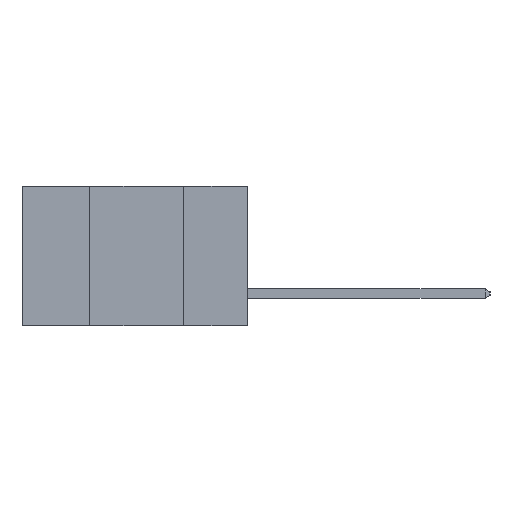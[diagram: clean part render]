
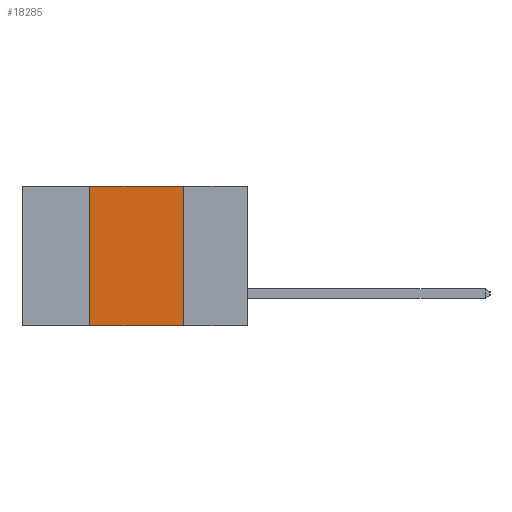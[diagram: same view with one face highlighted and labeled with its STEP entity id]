
A CAD part, left-side view. The second image highlights one B-rep face of the part: STEP entity #18285.
In plain terms, the highlighted planar face has unit normal (-1, 0, 0).
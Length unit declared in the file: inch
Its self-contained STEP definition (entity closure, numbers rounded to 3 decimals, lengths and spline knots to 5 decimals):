
#1420 = VERTEX_POINT ( 'NONE', #10792 ) ;
#1421 = CARTESIAN_POINT ( 'NONE',  ( 0., 0.42, 0. ) ) ;
#1899 = CARTESIAN_POINT ( 'NONE',  ( 0., 0.17, 0. ) ) ;
#2328 = EDGE_CURVE ( 'NONE', #19285, #11708, #9535, .T. ) ;
#3021 = AXIS2_PLACEMENT_3D ( 'NONE', #13472, #15572, #3329 ) ;
#3329 = DIRECTION ( 'NONE',  ( 0., 0., -1. ) ) ;
#4172 = VECTOR ( 'NONE', #22159, 39.37008 ) ;
#4933 = CARTESIAN_POINT ( 'NONE',  ( 0., 0.17, 0. ) ) ;
#5813 = FACE_OUTER_BOUND ( 'NONE', #22244, .T. ) ;
#6110 = VECTOR ( 'NONE', #19828, 39.37008 ) ;
#7272 = CARTESIAN_POINT ( 'NONE',  ( 0., 0.42, 0. ) ) ;
#9337 = DIRECTION ( 'NONE',  ( 0., 0., 1. ) ) ;
#9535 = LINE ( 'NONE', #1899, #4172 ) ;
#10020 = LINE ( 'NONE', #26420, #14842 ) ;
#10792 = CARTESIAN_POINT ( 'NONE',  ( 0., 0.42, -0.37 ) ) ;
#11410 = PLANE ( 'NONE',  #3021 ) ;
#11708 = VERTEX_POINT ( 'NONE', #19326 ) ;
#12136 = DIRECTION ( 'NONE',  ( 0., -1., 0. ) ) ;
#12950 = ORIENTED_EDGE ( 'NONE', *, *, #16760, .F. ) ;
#13000 = LINE ( 'NONE', #7272, #23277 ) ;
#13472 = CARTESIAN_POINT ( 'NONE',  ( 0., 0.6, 0. ) ) ;
#14244 = ORIENTED_EDGE ( 'NONE', *, *, #26061, .F. ) ;
#14842 = VECTOR ( 'NONE', #12136, 39.37008 ) ;
#15572 = DIRECTION ( 'NONE',  ( 1., 0., 0. ) ) ;
#16760 = EDGE_CURVE ( 'NONE', #24288, #19285, #10020, .T. ) ;
#16925 = ORIENTED_EDGE ( 'NONE', *, *, #22009, .T. ) ;
#17790 = CARTESIAN_POINT ( 'NONE',  ( 0., 0.6, -0.37 ) ) ;
#18285 = ADVANCED_FACE ( 'NONE', ( #5813 ), #11410, .F. ) ;
#19285 = VERTEX_POINT ( 'NONE', #4933 ) ;
#19326 = CARTESIAN_POINT ( 'NONE',  ( 0., 0.17, -0.37 ) ) ;
#19828 = DIRECTION ( 'NONE',  ( 0., -1., 0. ) ) ;
#22009 = EDGE_CURVE ( 'NONE', #1420, #11708, #22423, .T. ) ;
#22159 = DIRECTION ( 'NONE',  ( 0., 0., -1. ) ) ;
#22244 = EDGE_LOOP ( 'NONE', ( #23483, #12950, #14244, #16925 ) ) ;
#22423 = LINE ( 'NONE', #17790, #6110 ) ;
#23277 = VECTOR ( 'NONE', #9337, 39.37008 ) ;
#23483 = ORIENTED_EDGE ( 'NONE', *, *, #2328, .F. ) ;
#24288 = VERTEX_POINT ( 'NONE', #1421 ) ;
#26061 = EDGE_CURVE ( 'NONE', #1420, #24288, #13000, .T. ) ;
#26420 = CARTESIAN_POINT ( 'NONE',  ( 0., 0.6, 0. ) ) ;
